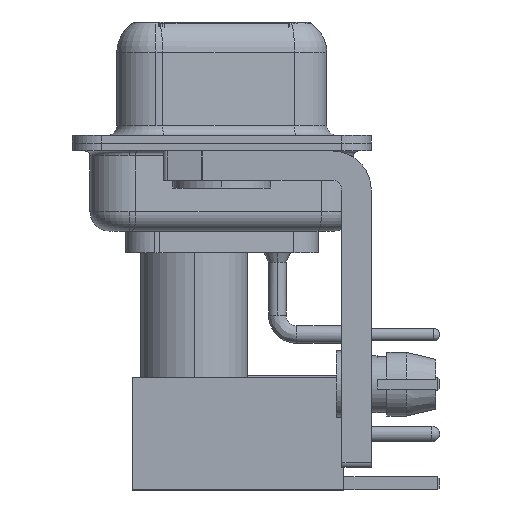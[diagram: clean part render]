
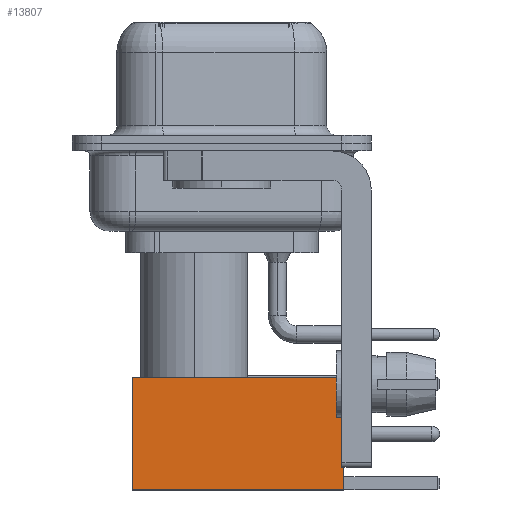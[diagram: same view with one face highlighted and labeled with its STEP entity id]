
A CAD part, left-side view. The second image highlights one B-rep face of the part: STEP entity #13807.
In plain terms, the highlighted face is planar.
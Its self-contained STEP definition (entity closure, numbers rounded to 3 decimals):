
#2346 = EDGE_CURVE ( 'NONE', #10226, #28712, #7008, .T. ) ;
#2404 = CARTESIAN_POINT ( 'NONE',  ( 2.875, 2.875, 0. ) ) ;
#3803 = CARTESIAN_POINT ( 'NONE',  ( 0., 2.875, 0. ) ) ;
#7008 = LINE ( 'NONE', #30444, #21851 ) ;
#7521 = AXIS2_PLACEMENT_3D ( 'NONE', #20132, #8502, #31965 ) ;
#7551 = EDGE_CURVE ( 'NONE', #32934, #20618, #16070, .T. ) ;
#8502 = DIRECTION ( 'NONE',  ( 0., 1., 0. ) ) ;
#9774 = EDGE_LOOP ( 'NONE', ( #28611, #17654, #24723, #18181 ) ) ;
#9786 = DIRECTION ( 'NONE',  ( -1., 0., 0. ) ) ;
#10226 = VERTEX_POINT ( 'NONE', #18696 ) ;
#10307 = CARTESIAN_POINT ( 'NONE',  ( -2.875, 2.875, 0. ) ) ;
#11503 = VECTOR ( 'NONE', #24360, 1000. ) ;
#13807 = ADVANCED_FACE ( 'NONE', ( #29211 ), #14132, .T. ) ;
#14132 = PLANE ( 'NONE',  #7521 ) ;
#14608 = VECTOR ( 'NONE', #21108, 1000. ) ;
#16070 = LINE ( 'NONE', #30414, #14608 ) ;
#17654 = ORIENTED_EDGE ( 'NONE', *, *, #30205, .T. ) ;
#18181 = ORIENTED_EDGE ( 'NONE', *, *, #21394, .F. ) ;
#18696 = CARTESIAN_POINT ( 'NONE',  ( -2.875, 2.875, 10.82 ) ) ;
#18764 = CARTESIAN_POINT ( 'NONE',  ( 0., 2.875, 10.82 ) ) ;
#20132 = CARTESIAN_POINT ( 'NONE',  ( 2.875, 2.875, 0. ) ) ;
#20618 = VERTEX_POINT ( 'NONE', #2404 ) ;
#21108 = DIRECTION ( 'NONE',  ( 0., 0., -1. ) ) ;
#21394 = EDGE_CURVE ( 'NONE', #32934, #10226, #30206, .T. ) ;
#21851 = VECTOR ( 'NONE', #30067, 1000. ) ;
#24360 = DIRECTION ( 'NONE',  ( -1., 0., 0. ) ) ;
#24649 = LINE ( 'NONE', #3803, #29751 ) ;
#24723 = ORIENTED_EDGE ( 'NONE', *, *, #2346, .F. ) ;
#27506 = CARTESIAN_POINT ( 'NONE',  ( 2.875, 2.875, 10.82 ) ) ;
#28611 = ORIENTED_EDGE ( 'NONE', *, *, #7551, .T. ) ;
#28712 = VERTEX_POINT ( 'NONE', #10307 ) ;
#29211 = FACE_OUTER_BOUND ( 'NONE', #9774, .T. ) ;
#29751 = VECTOR ( 'NONE', #9786, 1000. ) ;
#30067 = DIRECTION ( 'NONE',  ( 0., 0., -1. ) ) ;
#30205 = EDGE_CURVE ( 'NONE', #20618, #28712, #24649, .T. ) ;
#30206 = LINE ( 'NONE', #18764, #11503 ) ;
#30414 = CARTESIAN_POINT ( 'NONE',  ( 2.875, 2.875, 0. ) ) ;
#30444 = CARTESIAN_POINT ( 'NONE',  ( -2.875, 2.875, 0. ) ) ;
#31965 = DIRECTION ( 'NONE',  ( 0., 0., 1. ) ) ;
#32934 = VERTEX_POINT ( 'NONE', #27506 ) ;
